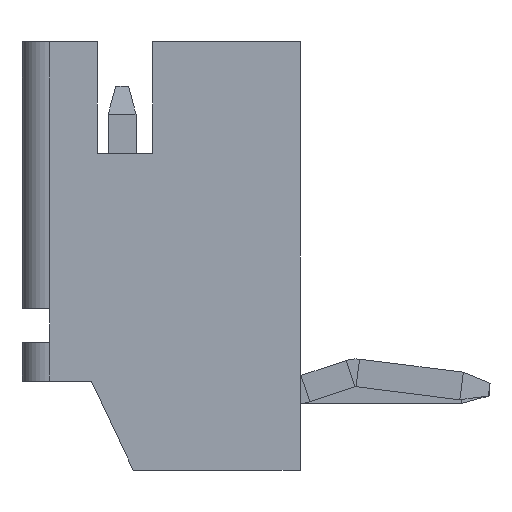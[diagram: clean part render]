
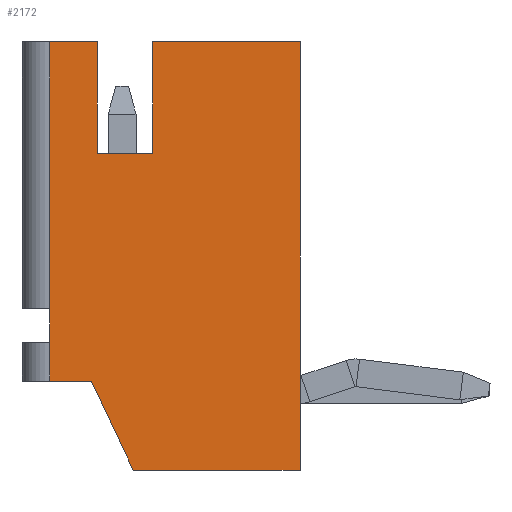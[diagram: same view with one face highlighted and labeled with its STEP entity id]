
A CAD part, left-side view. The second image highlights one B-rep face of the part: STEP entity #2172.
In plain terms, the highlighted planar face has unit normal (-1, 0, 0).
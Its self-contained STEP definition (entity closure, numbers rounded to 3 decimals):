
#6 = FACE_OUTER_BOUND ( 'NONE', #3257, .T. ) ;
#24 = DIRECTION ( 'NONE',  ( 0., -0.424, -0.905 ) ) ;
#226 = LINE ( 'NONE', #4507, #6372 ) ;
#250 = EDGE_CURVE ( 'NONE', #5063, #3990, #226, .T. ) ;
#475 = EDGE_CURVE ( 'NONE', #5428, #2713, #1490, .T. ) ;
#488 = VERTEX_POINT ( 'NONE', #5570 ) ;
#554 = CARTESIAN_POINT ( 'NONE',  ( -2., -3.2, 6.1 ) ) ;
#710 = EDGE_CURVE ( 'NONE', #2713, #2862, #2056, .T. ) ;
#787 = CARTESIAN_POINT ( 'NONE',  ( -2., 0.45, 4.1 ) ) ;
#931 = CARTESIAN_POINT ( 'NONE',  ( -2., 1.3, 0.7 ) ) ;
#945 = EDGE_CURVE ( 'NONE', #5439, #2776, #4171, .T. ) ;
#1335 = DIRECTION ( 'NONE',  ( 0., 1., 0. ) ) ;
#1484 = DIRECTION ( 'NONE',  ( -1., 0., 0. ) ) ;
#1490 = LINE ( 'NONE', #5479, #4178 ) ;
#1508 = DIRECTION ( 'NONE',  ( 0., -1., 0. ) ) ;
#1937 = VECTOR ( 'NONE', #5943, 1000. ) ;
#1975 = VECTOR ( 'NONE', #6008, 1000. ) ;
#1986 = ORIENTED_EDGE ( 'NONE', *, *, #475, .T. ) ;
#2015 = VECTOR ( 'NONE', #1335, 1000. ) ;
#2056 = LINE ( 'NONE', #6791, #3908 ) ;
#2139 = CARTESIAN_POINT ( 'NONE',  ( -2., 1.3, 1.3 ) ) ;
#2172 = ADVANCED_FACE ( 'NONE', ( #6 ), #6926, .T. ) ;
#2184 = ORIENTED_EDGE ( 'NONE', *, *, #945, .T. ) ;
#2185 = LINE ( 'NONE', #6273, #4377 ) ;
#2256 = ORIENTED_EDGE ( 'NONE', *, *, #6763, .T. ) ;
#2365 = DIRECTION ( 'NONE',  ( 0., 0., 1. ) ) ;
#2378 = ORIENTED_EDGE ( 'NONE', *, *, #6846, .T. ) ;
#2579 = LINE ( 'NONE', #6032, #2658 ) ;
#2655 = ORIENTED_EDGE ( 'NONE', *, *, #250, .T. ) ;
#2658 = VECTOR ( 'NONE', #3818, 1000. ) ;
#2713 = VERTEX_POINT ( 'NONE', #5195 ) ;
#2776 = VERTEX_POINT ( 'NONE', #6805 ) ;
#2862 = VERTEX_POINT ( 'NONE', #4642 ) ;
#2941 = VERTEX_POINT ( 'NONE', #2976 ) ;
#2976 = CARTESIAN_POINT ( 'NONE',  ( -2., -0.55, 6.1 ) ) ;
#3021 = VECTOR ( 'NONE', #24, 1000. ) ;
#3156 = EDGE_CURVE ( 'NONE', #488, #6529, #3292, .T. ) ;
#3257 = EDGE_LOOP ( 'NONE', ( #6484, #1986, #4472, #5180, #2184, #6207, #5201, #5151, #2378, #2655, #2256, #4365 ) ) ;
#3264 = VECTOR ( 'NONE', #5894, 1000. ) ;
#3292 = LINE ( 'NONE', #5632, #3536 ) ;
#3536 = VECTOR ( 'NONE', #5601, 1000. ) ;
#3551 = DIRECTION ( 'NONE',  ( 0., 1., 0. ) ) ;
#3617 = LINE ( 'NONE', #5616, #2015 ) ;
#3628 = EDGE_CURVE ( 'NONE', #2862, #5439, #3781, .T. ) ;
#3660 = CARTESIAN_POINT ( 'NONE',  ( -2., -3.2, 6.1 ) ) ;
#3661 = EDGE_CURVE ( 'NONE', #6529, #5428, #5636, .T. ) ;
#3781 = LINE ( 'NONE', #3836, #3021 ) ;
#3806 = EDGE_CURVE ( 'NONE', #2941, #5898, #4449, .T. ) ;
#3818 = DIRECTION ( 'NONE',  ( 0., 1., 0. ) ) ;
#3836 = CARTESIAN_POINT ( 'NONE',  ( -2., -0.2, -1.6 ) ) ;
#3908 = VECTOR ( 'NONE', #4671, 1000. ) ;
#3990 = VERTEX_POINT ( 'NONE', #5247 ) ;
#4171 = LINE ( 'NONE', #4466, #1975 ) ;
#4178 = VECTOR ( 'NONE', #6104, 1000. ) ;
#4247 = EDGE_CURVE ( 'NONE', #5396, #2941, #2579, .T. ) ;
#4310 = CARTESIAN_POINT ( 'NONE',  ( -2., -0.2, -1.6 ) ) ;
#4365 = ORIENTED_EDGE ( 'NONE', *, *, #3156, .T. ) ;
#4377 = VECTOR ( 'NONE', #3551, 1000. ) ;
#4449 = LINE ( 'NONE', #6160, #6293 ) ;
#4466 = CARTESIAN_POINT ( 'NONE',  ( -2., -3.2, -1.6 ) ) ;
#4472 = ORIENTED_EDGE ( 'NONE', *, *, #710, .T. ) ;
#4507 = CARTESIAN_POINT ( 'NONE',  ( -2., 0.45, 6.1 ) ) ;
#4642 = CARTESIAN_POINT ( 'NONE',  ( -2., 0.55, 0. ) ) ;
#4671 = DIRECTION ( 'NONE',  ( 0., -1., 0. ) ) ;
#4710 = CARTESIAN_POINT ( 'NONE',  ( -2., 0., 0. ) ) ;
#4799 = EDGE_CURVE ( 'NONE', #2776, #5396, #4866, .T. ) ;
#4866 = LINE ( 'NONE', #554, #3264 ) ;
#4877 = AXIS2_PLACEMENT_3D ( 'NONE', #4710, #1484, #1508 ) ;
#5063 = VERTEX_POINT ( 'NONE', #787 ) ;
#5151 = ORIENTED_EDGE ( 'NONE', *, *, #3806, .T. ) ;
#5153 = DIRECTION ( 'NONE',  ( 0., 0., -1. ) ) ;
#5180 = ORIENTED_EDGE ( 'NONE', *, *, #3628, .T. ) ;
#5195 = CARTESIAN_POINT ( 'NONE',  ( -2., 1.3, 0. ) ) ;
#5201 = ORIENTED_EDGE ( 'NONE', *, *, #4247, .T. ) ;
#5247 = CARTESIAN_POINT ( 'NONE',  ( -2., 0.45, 6.1 ) ) ;
#5396 = VERTEX_POINT ( 'NONE', #3660 ) ;
#5428 = VERTEX_POINT ( 'NONE', #931 ) ;
#5439 = VERTEX_POINT ( 'NONE', #4310 ) ;
#5479 = CARTESIAN_POINT ( 'NONE',  ( -2., 1.3, 0. ) ) ;
#5570 = CARTESIAN_POINT ( 'NONE',  ( -2., 1.3, 6.1 ) ) ;
#5601 = DIRECTION ( 'NONE',  ( 0., 0., -1. ) ) ;
#5616 = CARTESIAN_POINT ( 'NONE',  ( -2., 1.8, 6.1 ) ) ;
#5632 = CARTESIAN_POINT ( 'NONE',  ( -2., 1.3, 0. ) ) ;
#5636 = LINE ( 'NONE', #5924, #1937 ) ;
#5894 = DIRECTION ( 'NONE',  ( 0., 0., 1. ) ) ;
#5898 = VERTEX_POINT ( 'NONE', #6942 ) ;
#5924 = CARTESIAN_POINT ( 'NONE',  ( -2., 1.3, 1.3 ) ) ;
#5943 = DIRECTION ( 'NONE',  ( 0., 0., -1. ) ) ;
#6008 = DIRECTION ( 'NONE',  ( 0., -1., 0. ) ) ;
#6032 = CARTESIAN_POINT ( 'NONE',  ( -2., -0.55, 6.1 ) ) ;
#6104 = DIRECTION ( 'NONE',  ( 0., 0., -1. ) ) ;
#6160 = CARTESIAN_POINT ( 'NONE',  ( -2., -0.55, 6.1 ) ) ;
#6207 = ORIENTED_EDGE ( 'NONE', *, *, #4799, .T. ) ;
#6273 = CARTESIAN_POINT ( 'NONE',  ( -2., 0.45, 4.1 ) ) ;
#6293 = VECTOR ( 'NONE', #5153, 1000. ) ;
#6372 = VECTOR ( 'NONE', #2365, 1000. ) ;
#6484 = ORIENTED_EDGE ( 'NONE', *, *, #3661, .T. ) ;
#6529 = VERTEX_POINT ( 'NONE', #2139 ) ;
#6763 = EDGE_CURVE ( 'NONE', #3990, #488, #3617, .T. ) ;
#6791 = CARTESIAN_POINT ( 'NONE',  ( -2., 1.8, 0. ) ) ;
#6805 = CARTESIAN_POINT ( 'NONE',  ( -2., -3.2, -1.6 ) ) ;
#6846 = EDGE_CURVE ( 'NONE', #5898, #5063, #2185, .T. ) ;
#6926 = PLANE ( 'NONE',  #4877 ) ;
#6942 = CARTESIAN_POINT ( 'NONE',  ( -2., -0.55, 4.1 ) ) ;
